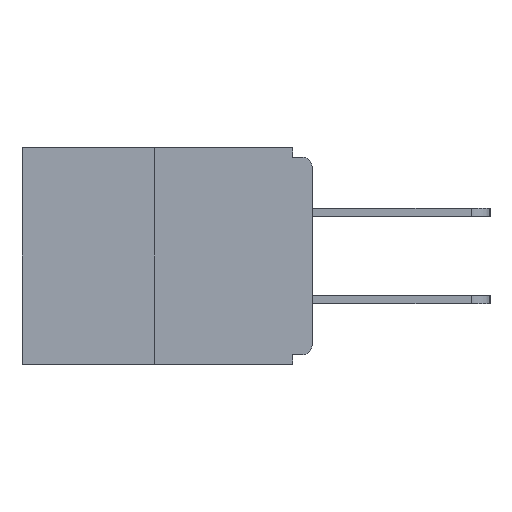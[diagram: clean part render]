
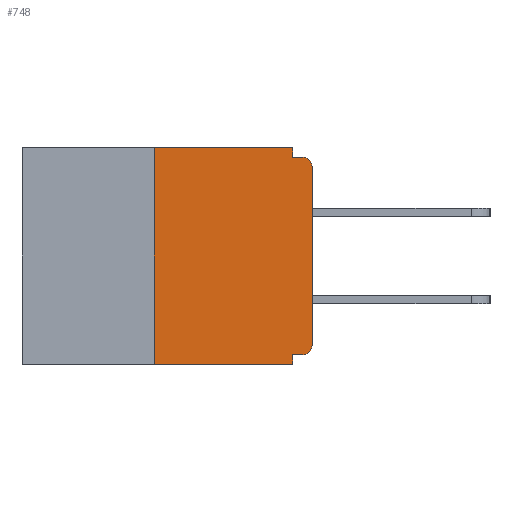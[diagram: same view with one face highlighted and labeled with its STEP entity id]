
A CAD part, left-side view. The second image highlights one B-rep face of the part: STEP entity #748.
In plain terms, the highlighted planar face has unit normal (-1, 0, 0).
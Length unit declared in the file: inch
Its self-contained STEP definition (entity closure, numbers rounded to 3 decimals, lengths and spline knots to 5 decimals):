
#75 = CARTESIAN_POINT ( 'NONE',  ( 0., 0.031, 0. ) ) ;
#263 = VERTEX_POINT ( 'NONE', #3487 ) ;
#356 = AXIS2_PLACEMENT_3D ( 'NONE', #10391, #4713, #9505 ) ;
#748 = ADVANCED_FACE ( 'NONE', ( #1924 ), #3024, .F. ) ;
#841 = CARTESIAN_POINT ( 'NONE',  ( 0., 0., -0.328 ) ) ;
#994 = VERTEX_POINT ( 'NONE', #75 ) ;
#1594 = VERTEX_POINT ( 'NONE', #10467 ) ;
#1834 = ORIENTED_EDGE ( 'NONE', *, *, #7152, .F. ) ;
#1924 = FACE_OUTER_BOUND ( 'NONE', #2826, .T. ) ;
#2341 = VECTOR ( 'NONE', #9443, 39.37008 ) ;
#2399 = DIRECTION ( 'NONE',  ( 0., 0., -1. ) ) ;
#2461 = AXIS2_PLACEMENT_3D ( 'NONE', #3796, #6685, #8740 ) ;
#2712 = VECTOR ( 'NONE', #4664, 39.37008 ) ;
#2826 = EDGE_LOOP ( 'NONE', ( #1834, #9327, #5102, #5253, #9999, #6551, #4480, #11839, #10759, #5661 ) ) ;
#2946 = CARTESIAN_POINT ( 'NONE',  ( 0., 0.25, 0. ) ) ;
#3024 = PLANE ( 'NONE',  #356 ) ;
#3472 = EDGE_CURVE ( 'NONE', #7416, #263, #8178, .T. ) ;
#3487 = CARTESIAN_POINT ( 'NONE',  ( 0., 0.015, -0.015 ) ) ;
#3488 = DIRECTION ( 'NONE',  ( 0., -1., 0. ) ) ;
#3705 = VECTOR ( 'NONE', #11031, 39.37008 ) ;
#3756 = VECTOR ( 'NONE', #7256, 39.37008 ) ;
#3796 = CARTESIAN_POINT ( 'NONE',  ( 0., 0.015, -0.313 ) ) ;
#3875 = DIRECTION ( 'NONE',  ( 0., 0., -1. ) ) ;
#4061 = LINE ( 'NONE', #10535, #7778 ) ;
#4371 = LINE ( 'NONE', #841, #3756 ) ;
#4480 = ORIENTED_EDGE ( 'NONE', *, *, #4761, .T. ) ;
#4664 = DIRECTION ( 'NONE',  ( 0., -1., 0. ) ) ;
#4713 = DIRECTION ( 'NONE',  ( 1., 0., 0. ) ) ;
#4761 = EDGE_CURVE ( 'NONE', #9867, #5853, #7515, .T. ) ;
#4993 = VERTEX_POINT ( 'NONE', #11645 ) ;
#5102 = ORIENTED_EDGE ( 'NONE', *, *, #8430, .T. ) ;
#5253 = ORIENTED_EDGE ( 'NONE', *, *, #11168, .F. ) ;
#5313 = EDGE_CURVE ( 'NONE', #5853, #263, #6078, .T. ) ;
#5469 = CARTESIAN_POINT ( 'NONE',  ( 0., 0., -0.03 ) ) ;
#5661 = ORIENTED_EDGE ( 'NONE', *, *, #8228, .F. ) ;
#5761 = EDGE_CURVE ( 'NONE', #10544, #1594, #4371, .T. ) ;
#5792 = LINE ( 'NONE', #2946, #9403 ) ;
#5853 = VERTEX_POINT ( 'NONE', #5469 ) ;
#6078 = CIRCLE ( 'NONE', #6684, 0.015 ) ;
#6319 = CARTESIAN_POINT ( 'NONE',  ( 0., 0., -0.313 ) ) ;
#6551 = ORIENTED_EDGE ( 'NONE', *, *, #11562, .T. ) ;
#6684 = AXIS2_PLACEMENT_3D ( 'NONE', #7894, #10053, #2399 ) ;
#6685 = DIRECTION ( 'NONE',  ( -1., 0., 0. ) ) ;
#6722 = VERTEX_POINT ( 'NONE', #7190 ) ;
#6970 = VECTOR ( 'NONE', #3488, 39.37008 ) ;
#6979 = CIRCLE ( 'NONE', #2461, 0.015 ) ;
#7152 = EDGE_CURVE ( 'NONE', #4993, #994, #11888, .T. ) ;
#7190 = CARTESIAN_POINT ( 'NONE',  ( 0., 0.031, -0.343 ) ) ;
#7253 = DIRECTION ( 'NONE',  ( 0., 0., 1. ) ) ;
#7256 = DIRECTION ( 'NONE',  ( 0., 1., 0. ) ) ;
#7416 = VERTEX_POINT ( 'NONE', #7751 ) ;
#7515 = LINE ( 'NONE', #9467, #9882 ) ;
#7678 = LINE ( 'NONE', #9636, #2341 ) ;
#7751 = CARTESIAN_POINT ( 'NONE',  ( 0., 0.031, -0.015 ) ) ;
#7778 = VECTOR ( 'NONE', #3875, 39.37008 ) ;
#7894 = CARTESIAN_POINT ( 'NONE',  ( 0., 0.015, -0.03 ) ) ;
#8178 = LINE ( 'NONE', #10958, #6970 ) ;
#8182 = CARTESIAN_POINT ( 'NONE',  ( 0., 0.031, 0. ) ) ;
#8228 = EDGE_CURVE ( 'NONE', #994, #7416, #10097, .T. ) ;
#8430 = EDGE_CURVE ( 'NONE', #11431, #6722, #7678, .T. ) ;
#8486 = CARTESIAN_POINT ( 'NONE',  ( 0., 0.46, 0. ) ) ;
#8740 = DIRECTION ( 'NONE',  ( 0., 0., -1. ) ) ;
#9327 = ORIENTED_EDGE ( 'NONE', *, *, #9428, .F. ) ;
#9403 = VECTOR ( 'NONE', #9608, 39.37008 ) ;
#9428 = EDGE_CURVE ( 'NONE', #11431, #4993, #5792, .T. ) ;
#9443 = DIRECTION ( 'NONE',  ( 0., -1., 0. ) ) ;
#9467 = CARTESIAN_POINT ( 'NONE',  ( 0., 0., 0. ) ) ;
#9505 = DIRECTION ( 'NONE',  ( 0., 0., -1. ) ) ;
#9608 = DIRECTION ( 'NONE',  ( 0., 0., 1. ) ) ;
#9636 = CARTESIAN_POINT ( 'NONE',  ( 0., 0.46, -0.343 ) ) ;
#9867 = VERTEX_POINT ( 'NONE', #6319 ) ;
#9882 = VECTOR ( 'NONE', #7253, 39.37008 ) ;
#9999 = ORIENTED_EDGE ( 'NONE', *, *, #5761, .F. ) ;
#10053 = DIRECTION ( 'NONE',  ( -1., 0., 0. ) ) ;
#10097 = LINE ( 'NONE', #8182, #3705 ) ;
#10102 = CARTESIAN_POINT ( 'NONE',  ( 0., 0.25, -0.343 ) ) ;
#10391 = CARTESIAN_POINT ( 'NONE',  ( 0., 0.46, 0. ) ) ;
#10467 = CARTESIAN_POINT ( 'NONE',  ( 0., 0.031, -0.328 ) ) ;
#10535 = CARTESIAN_POINT ( 'NONE',  ( 0., 0.031, -0.343 ) ) ;
#10544 = VERTEX_POINT ( 'NONE', #10938 ) ;
#10759 = ORIENTED_EDGE ( 'NONE', *, *, #3472, .F. ) ;
#10938 = CARTESIAN_POINT ( 'NONE',  ( 0., 0.015, -0.328 ) ) ;
#10958 = CARTESIAN_POINT ( 'NONE',  ( 0., 0., -0.015 ) ) ;
#11031 = DIRECTION ( 'NONE',  ( 0., 0., -1. ) ) ;
#11168 = EDGE_CURVE ( 'NONE', #1594, #6722, #4061, .T. ) ;
#11431 = VERTEX_POINT ( 'NONE', #10102 ) ;
#11562 = EDGE_CURVE ( 'NONE', #10544, #9867, #6979, .T. ) ;
#11645 = CARTESIAN_POINT ( 'NONE',  ( 0., 0.25, 0. ) ) ;
#11839 = ORIENTED_EDGE ( 'NONE', *, *, #5313, .T. ) ;
#11888 = LINE ( 'NONE', #8486, #2712 ) ;
